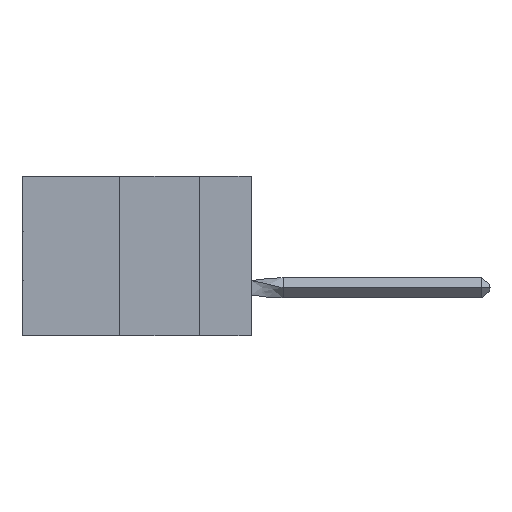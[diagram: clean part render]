
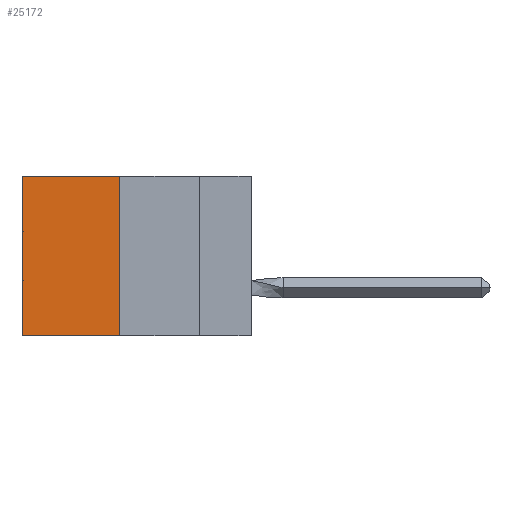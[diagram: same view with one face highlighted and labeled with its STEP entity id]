
A CAD part, left-side view. The second image highlights one B-rep face of the part: STEP entity #25172.
In plain terms, the highlighted planar face has unit normal (-1, 0, 0).
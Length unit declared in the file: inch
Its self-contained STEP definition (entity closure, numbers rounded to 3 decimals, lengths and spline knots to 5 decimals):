
#1005 = EDGE_LOOP ( 'NONE', ( #7605, #36684, #29171, #29492 ) ) ;
#5574 = CARTESIAN_POINT ( 'NONE',  ( 0.305, 0.413, 0. ) ) ;
#6174 = DIRECTION ( 'NONE',  ( 0., 0., -1. ) ) ;
#6966 = EDGE_CURVE ( 'NONE', #30398, #32937, #20742, .T. ) ;
#7562 = FACE_OUTER_BOUND ( 'NONE', #1005, .T. ) ;
#7605 = ORIENTED_EDGE ( 'NONE', *, *, #42378, .T. ) ;
#8401 = CARTESIAN_POINT ( 'NONE',  ( 0.305, 0.413, -0.5 ) ) ;
#9346 = LINE ( 'NONE', #25220, #26383 ) ;
#9516 = DIRECTION ( 'NONE',  ( 1., 0., 0. ) ) ;
#9536 = CARTESIAN_POINT ( 'NONE',  ( 0.305, 0.72, 0. ) ) ;
#15121 = VERTEX_POINT ( 'NONE', #5574 ) ;
#16202 = PLANE ( 'NONE',  #20124 ) ;
#19919 = CARTESIAN_POINT ( 'NONE',  ( 0.305, 0.413, -0.5 ) ) ;
#20124 = AXIS2_PLACEMENT_3D ( 'NONE', #19919, #9516, #6174 ) ;
#20569 = CARTESIAN_POINT ( 'NONE',  ( 0.305, 0.413, -0.5 ) ) ;
#20672 = LINE ( 'NONE', #32709, #38858 ) ;
#20742 = LINE ( 'NONE', #8401, #42150 ) ;
#25172 = ADVANCED_FACE ( 'NONE', ( #7562 ), #16202, .F. ) ;
#25220 = CARTESIAN_POINT ( 'NONE',  ( 0.305, 0.413, -0.5 ) ) ;
#25641 = EDGE_CURVE ( 'NONE', #15121, #37603, #33161, .T. ) ;
#26383 = VECTOR ( 'NONE', #29235, 39.37008 ) ;
#29171 = ORIENTED_EDGE ( 'NONE', *, *, #30092, .F. ) ;
#29235 = DIRECTION ( 'NONE',  ( 0., 0., -1. ) ) ;
#29492 = ORIENTED_EDGE ( 'NONE', *, *, #25641, .T. ) ;
#30092 = EDGE_CURVE ( 'NONE', #15121, #30398, #9346, .T. ) ;
#30398 = VERTEX_POINT ( 'NONE', #20569 ) ;
#31842 = DIRECTION ( 'NONE',  ( 0., 1., 0. ) ) ;
#32550 = DIRECTION ( 'NONE',  ( 0., 0., -1. ) ) ;
#32709 = CARTESIAN_POINT ( 'NONE',  ( 0.305, 0.72, -0.5 ) ) ;
#32937 = VERTEX_POINT ( 'NONE', #41915 ) ;
#33161 = LINE ( 'NONE', #43624, #43861 ) ;
#36684 = ORIENTED_EDGE ( 'NONE', *, *, #6966, .F. ) ;
#36767 = DIRECTION ( 'NONE',  ( 0., 1., 0. ) ) ;
#37603 = VERTEX_POINT ( 'NONE', #9536 ) ;
#38858 = VECTOR ( 'NONE', #32550, 39.37008 ) ;
#41915 = CARTESIAN_POINT ( 'NONE',  ( 0.305, 0.72, -0.5 ) ) ;
#42150 = VECTOR ( 'NONE', #31842, 39.37008 ) ;
#42378 = EDGE_CURVE ( 'NONE', #37603, #32937, #20672, .T. ) ;
#43624 = CARTESIAN_POINT ( 'NONE',  ( 0.305, 0.413, 0. ) ) ;
#43861 = VECTOR ( 'NONE', #36767, 39.37008 ) ;
